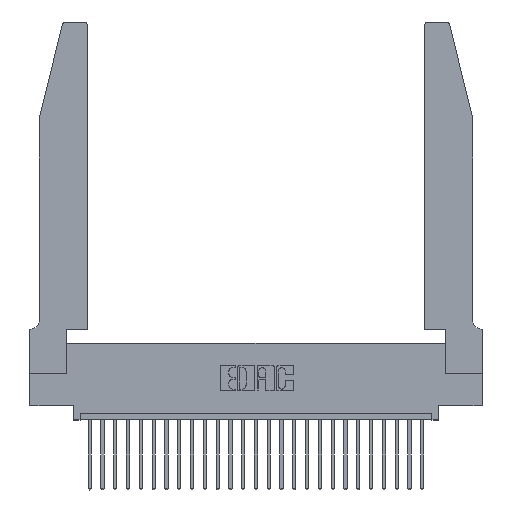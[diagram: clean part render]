
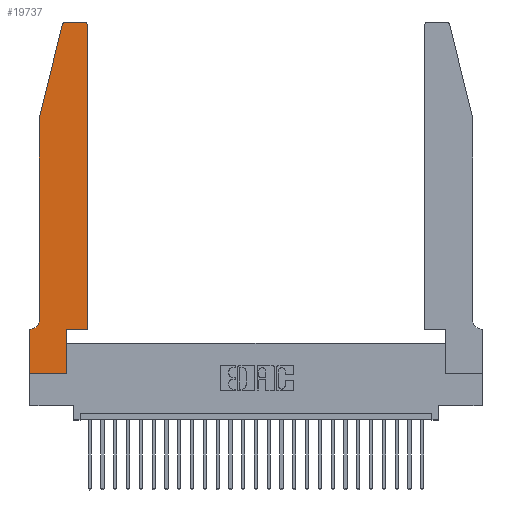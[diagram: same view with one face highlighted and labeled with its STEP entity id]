
A CAD part, top view. The second image highlights one B-rep face of the part: STEP entity #19737.
In plain terms, the highlighted planar face has unit normal (0, 0, 1).
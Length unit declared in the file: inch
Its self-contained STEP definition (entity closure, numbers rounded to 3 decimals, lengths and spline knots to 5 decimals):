
#3 = ORIENTED_EDGE ( 'NONE', *, *, #10324, .T. ) ;
#99 = ORIENTED_EDGE ( 'NONE', *, *, #11637, .T. ) ;
#310 = VECTOR ( 'NONE', #26997, 39.37008 ) ;
#587 = CARTESIAN_POINT ( 'NONE',  ( 0.4505, 0.35, 0.37 ) ) ;
#595 = VERTEX_POINT ( 'NONE', #23896 ) ;
#774 = CARTESIAN_POINT ( 'NONE',  ( 0.0755, 2., 0.37 ) ) ;
#916 = ORIENTED_EDGE ( 'NONE', *, *, #18882, .T. ) ;
#926 = VECTOR ( 'NONE', #8713, 39.37008 ) ;
#1210 = LINE ( 'NONE', #774, #2529 ) ;
#1296 = PLANE ( 'NONE',  #19410 ) ;
#1666 = DIRECTION ( 'NONE',  ( 0., 0., 1. ) ) ;
#1791 = EDGE_CURVE ( 'NONE', #25378, #3455, #17079, .T. ) ;
#1840 = LINE ( 'NONE', #12017, #23540 ) ;
#1950 = CARTESIAN_POINT ( 'NONE',  ( 0., 0.35, 0.37 ) ) ;
#2055 = CARTESIAN_POINT ( 'NONE',  ( 0., 0., 0.37 ) ) ;
#2126 = CARTESIAN_POINT ( 'NONE',  ( 0.4205, 2.75, 0.37 ) ) ;
#2213 = LINE ( 'NONE', #2055, #15659 ) ;
#2293 = ORIENTED_EDGE ( 'NONE', *, *, #18635, .T. ) ;
#2435 = DIRECTION ( 'NONE',  ( 0., 0., -1. ) ) ;
#2529 = VECTOR ( 'NONE', #17305, 39.37008 ) ;
#2637 = EDGE_CURVE ( 'NONE', #22454, #12547, #14750, .T. ) ;
#2896 = CARTESIAN_POINT ( 'NONE',  ( 0.0055, 0.42, 0.37 ) ) ;
#3312 = DIRECTION ( 'NONE',  ( 1., 0., 0. ) ) ;
#3455 = VERTEX_POINT ( 'NONE', #2126 ) ;
#3777 = DIRECTION ( 'NONE',  ( -1., 0., 0. ) ) ;
#3989 = EDGE_CURVE ( 'NONE', #595, #22454, #2213, .T. ) ;
#4068 = EDGE_CURVE ( 'NONE', #16335, #17943, #1210, .T. ) ;
#4543 = CARTESIAN_POINT ( 'NONE',  ( 0., 0., 0.37 ) ) ;
#4674 = VECTOR ( 'NONE', #6073, 39.37008 ) ;
#5113 = ORIENTED_EDGE ( 'NONE', *, *, #16507, .T. ) ;
#5473 = VERTEX_POINT ( 'NONE', #12301 ) ;
#5694 = CARTESIAN_POINT ( 'NONE',  ( 0.0755, 2., 0.37 ) ) ;
#6073 = DIRECTION ( 'NONE',  ( 1., 0., 0. ) ) ;
#7266 = CARTESIAN_POINT ( 'NONE',  ( 0.0755, 2., 0.37 ) ) ;
#7907 = CARTESIAN_POINT ( 'NONE',  ( 0.2865, 0.35, 0.37 ) ) ;
#8349 = ORIENTED_EDGE ( 'NONE', *, *, #12442, .T. ) ;
#8502 = CARTESIAN_POINT ( 'NONE',  ( 0.0755, 0.42, 0.37 ) ) ;
#8713 = DIRECTION ( 'NONE',  ( 0., 1., 0. ) ) ;
#9378 = DIRECTION ( 'NONE',  ( -1., 0., 0. ) ) ;
#10072 = LINE ( 'NONE', #17274, #926 ) ;
#10324 = EDGE_CURVE ( 'NONE', #10920, #5473, #21961, .T. ) ;
#10434 = DIRECTION ( 'NONE',  ( 1., 0., 0. ) ) ;
#10566 = LINE ( 'NONE', #15290, #20808 ) ;
#10752 = DIRECTION ( 'NONE',  ( 0., -1., 0. ) ) ;
#10875 = LINE ( 'NONE', #587, #4674 ) ;
#10920 = VERTEX_POINT ( 'NONE', #21885 ) ;
#11579 = CARTESIAN_POINT ( 'NONE',  ( 0.2865, 0.35, 0.37 ) ) ;
#11637 = EDGE_CURVE ( 'NONE', #20069, #595, #18583, .T. ) ;
#11737 = VECTOR ( 'NONE', #24280, 39.37008 ) ;
#11818 = CARTESIAN_POINT ( 'NONE',  ( 0.284, 2.72, 0.37 ) ) ;
#12017 = CARTESIAN_POINT ( 'NONE',  ( 0.2605, 2.75, 0.37 ) ) ;
#12301 = CARTESIAN_POINT ( 'NONE',  ( 0.25487, 2.72718, 0.37 ) ) ;
#12442 = EDGE_CURVE ( 'NONE', #22551, #20069, #10566, .T. ) ;
#12484 = CARTESIAN_POINT ( 'NONE',  ( 0.2865, 0., 0.37 ) ) ;
#12547 = VERTEX_POINT ( 'NONE', #11579 ) ;
#12831 = EDGE_CURVE ( 'NONE', #12547, #24909, #10875, .T. ) ;
#13430 = AXIS2_PLACEMENT_3D ( 'NONE', #2896, #2435, #9378 ) ;
#14311 = FACE_OUTER_BOUND ( 'NONE', #14540, .T. ) ;
#14504 = ORIENTED_EDGE ( 'NONE', *, *, #2637, .T. ) ;
#14540 = EDGE_LOOP ( 'NONE', ( #5113, #3, #2293, #22493, #21376, #8349, #99, #15085, #14504, #20896, #916, #17782 ) ) ;
#14750 = LINE ( 'NONE', #7907, #310 ) ;
#15085 = ORIENTED_EDGE ( 'NONE', *, *, #3989, .T. ) ;
#15290 = CARTESIAN_POINT ( 'NONE',  ( 0.0755, 0.35, 0.37 ) ) ;
#15659 = VECTOR ( 'NONE', #10434, 39.37008 ) ;
#16034 = CIRCLE ( 'NONE', #13430, 0.07 ) ;
#16335 = VERTEX_POINT ( 'NONE', #7266 ) ;
#16507 = EDGE_CURVE ( 'NONE', #3455, #10920, #1840, .T. ) ;
#16643 = CARTESIAN_POINT ( 'NONE',  ( 0.4505, 0.35, 0.37 ) ) ;
#17079 = CIRCLE ( 'NONE', #19918, 0.03 ) ;
#17274 = CARTESIAN_POINT ( 'NONE',  ( 0.4505, 0.35, 0.37 ) ) ;
#17305 = DIRECTION ( 'NONE',  ( 0., -1., 0. ) ) ;
#17782 = ORIENTED_EDGE ( 'NONE', *, *, #1791, .T. ) ;
#17943 = VERTEX_POINT ( 'NONE', #8502 ) ;
#18484 = EDGE_CURVE ( 'NONE', #17943, #22551, #16034, .T. ) ;
#18583 = LINE ( 'NONE', #4543, #24823 ) ;
#18635 = EDGE_CURVE ( 'NONE', #5473, #16335, #22954, .T. ) ;
#18882 = EDGE_CURVE ( 'NONE', #24909, #25378, #10072, .T. ) ;
#19339 = DIRECTION ( 'NONE',  ( -1., 0., 0. ) ) ;
#19410 = AXIS2_PLACEMENT_3D ( 'NONE', #24234, #26214, #3312 ) ;
#19737 = ADVANCED_FACE ( 'NONE', ( #14311 ), #1296, .T. ) ;
#19918 = AXIS2_PLACEMENT_3D ( 'NONE', #23462, #25562, #21245 ) ;
#20069 = VERTEX_POINT ( 'NONE', #1950 ) ;
#20808 = VECTOR ( 'NONE', #19339, 39.37008 ) ;
#20896 = ORIENTED_EDGE ( 'NONE', *, *, #12831, .T. ) ;
#21245 = DIRECTION ( 'NONE',  ( 1., 0., 0. ) ) ;
#21376 = ORIENTED_EDGE ( 'NONE', *, *, #18484, .T. ) ;
#21885 = CARTESIAN_POINT ( 'NONE',  ( 0.284, 2.75, 0.37 ) ) ;
#21961 = CIRCLE ( 'NONE', #24111, 0.03 ) ;
#22454 = VERTEX_POINT ( 'NONE', #12484 ) ;
#22493 = ORIENTED_EDGE ( 'NONE', *, *, #4068, .T. ) ;
#22551 = VERTEX_POINT ( 'NONE', #25754 ) ;
#22954 = LINE ( 'NONE', #5694, #11737 ) ;
#23462 = CARTESIAN_POINT ( 'NONE',  ( 0.4205, 2.72, 0.37 ) ) ;
#23540 = VECTOR ( 'NONE', #3777, 39.37008 ) ;
#23896 = CARTESIAN_POINT ( 'NONE',  ( 0., 0., 0.37 ) ) ;
#24111 = AXIS2_PLACEMENT_3D ( 'NONE', #11818, #1666, #26596 ) ;
#24153 = CARTESIAN_POINT ( 'NONE',  ( 0.4505, 2.72, 0.37 ) ) ;
#24234 = CARTESIAN_POINT ( 'NONE',  ( 0., 0.35, 0.37 ) ) ;
#24280 = DIRECTION ( 'NONE',  ( -0.239, -0.971, 0. ) ) ;
#24823 = VECTOR ( 'NONE', #10752, 39.37008 ) ;
#24909 = VERTEX_POINT ( 'NONE', #16643 ) ;
#25378 = VERTEX_POINT ( 'NONE', #24153 ) ;
#25562 = DIRECTION ( 'NONE',  ( 0., 0., 1. ) ) ;
#25754 = CARTESIAN_POINT ( 'NONE',  ( 0.0055, 0.35, 0.37 ) ) ;
#26214 = DIRECTION ( 'NONE',  ( 0., 0., 1. ) ) ;
#26596 = DIRECTION ( 'NONE',  ( 1., 0., 0. ) ) ;
#26997 = DIRECTION ( 'NONE',  ( 0., 1., 0. ) ) ;
